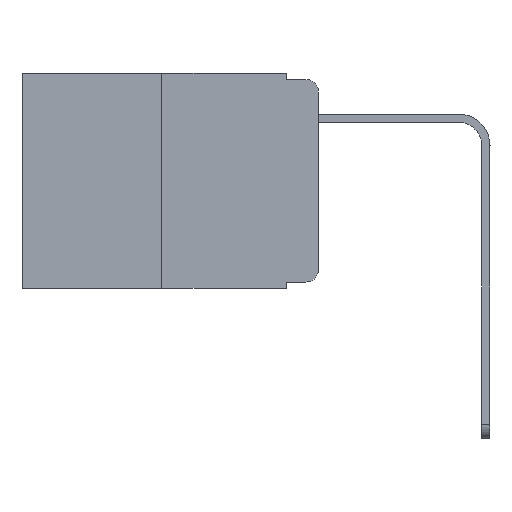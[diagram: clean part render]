
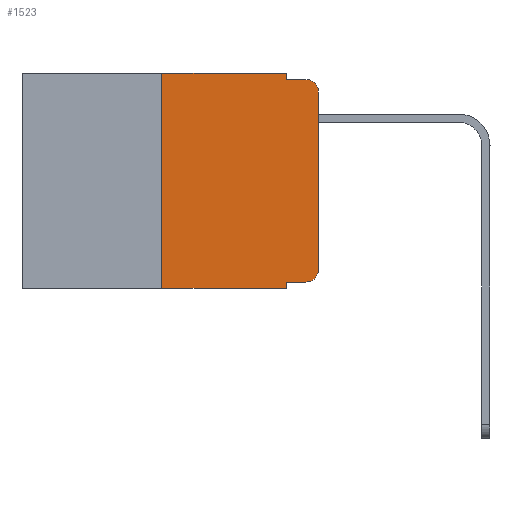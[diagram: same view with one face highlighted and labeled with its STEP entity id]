
A CAD part, left-side view. The second image highlights one B-rep face of the part: STEP entity #1523.
In plain terms, the highlighted planar face has unit normal (-1, 0, 0).
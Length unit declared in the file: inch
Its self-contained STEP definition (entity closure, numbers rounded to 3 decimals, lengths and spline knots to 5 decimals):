
#162 = CARTESIAN_POINT ( 'NONE',  ( 0., 0.473, 0. ) ) ;
#573 = CARTESIAN_POINT ( 'NONE',  ( 0., 0.473, -0.343 ) ) ;
#917 = EDGE_CURVE ( 'NONE', #14089, #12298, #3522, .T. ) ;
#1089 = VERTEX_POINT ( 'NONE', #14140 ) ;
#1265 = ORIENTED_EDGE ( 'NONE', *, *, #12177, .T. ) ;
#1493 = VERTEX_POINT ( 'NONE', #6013 ) ;
#1523 = ADVANCED_FACE ( 'NONE', ( #13903 ), #1693, .F. ) ;
#1693 = PLANE ( 'NONE',  #10979 ) ;
#1792 = CIRCLE ( 'NONE', #14482, 0.02 ) ;
#2038 = ORIENTED_EDGE ( 'NONE', *, *, #14747, .F. ) ;
#2066 = CARTESIAN_POINT ( 'NONE',  ( 0., 0.02, -0.313 ) ) ;
#2218 = VECTOR ( 'NONE', #8968, 39.37008 ) ;
#3108 = DIRECTION ( 'NONE',  ( 0., 0., -1. ) ) ;
#3147 = CARTESIAN_POINT ( 'NONE',  ( 0., 0.051, 0. ) ) ;
#3240 = DIRECTION ( 'NONE',  ( -1., 0., 0. ) ) ;
#3414 = VECTOR ( 'NONE', #8670, 39.37008 ) ;
#3522 = LINE ( 'NONE', #4336, #13734 ) ;
#3771 = LINE ( 'NONE', #573, #10218 ) ;
#3884 = VERTEX_POINT ( 'NONE', #7558 ) ;
#3907 = ORIENTED_EDGE ( 'NONE', *, *, #4260, .F. ) ;
#4260 = EDGE_CURVE ( 'NONE', #9914, #3884, #13710, .T. ) ;
#4336 = CARTESIAN_POINT ( 'NONE',  ( 0., 0., 0. ) ) ;
#4517 = DIRECTION ( 'NONE',  ( 0., 0., 1. ) ) ;
#5112 = LINE ( 'NONE', #3147, #7447 ) ;
#5507 = ORIENTED_EDGE ( 'NONE', *, *, #7386, .T. ) ;
#5905 = EDGE_CURVE ( 'NONE', #3884, #1493, #5112, .T. ) ;
#6013 = CARTESIAN_POINT ( 'NONE',  ( 0., 0.051, -0.01 ) ) ;
#6041 = CARTESIAN_POINT ( 'NONE',  ( 0., 0.25, 0. ) ) ;
#6193 = EDGE_CURVE ( 'NONE', #1493, #10311, #9038, .T. ) ;
#6269 = DIRECTION ( 'NONE',  ( -1., 0., 0. ) ) ;
#6521 = DIRECTION ( 'NONE',  ( 0., 0., -1. ) ) ;
#6540 = ORIENTED_EDGE ( 'NONE', *, *, #12832, .T. ) ;
#7133 = ORIENTED_EDGE ( 'NONE', *, *, #8048, .T. ) ;
#7386 = EDGE_CURVE ( 'NONE', #1089, #9643, #7921, .T. ) ;
#7447 = VECTOR ( 'NONE', #14461, 39.37008 ) ;
#7510 = CARTESIAN_POINT ( 'NONE',  ( 0., 0., -0.03 ) ) ;
#7558 = CARTESIAN_POINT ( 'NONE',  ( 0., 0.051, 0. ) ) ;
#7658 = CARTESIAN_POINT ( 'NONE',  ( 0., 0.051, -0.333 ) ) ;
#7764 = CARTESIAN_POINT ( 'NONE',  ( 0., 0.25, 0. ) ) ;
#7782 = VECTOR ( 'NONE', #9279, 39.37008 ) ;
#7921 = LINE ( 'NONE', #7658, #2218 ) ;
#8048 = EDGE_CURVE ( 'NONE', #9643, #14089, #14553, .T. ) ;
#8395 = CARTESIAN_POINT ( 'NONE',  ( 0., 0.25, -0.343 ) ) ;
#8418 = CARTESIAN_POINT ( 'NONE',  ( 0., 0.02, -0.01 ) ) ;
#8670 = DIRECTION ( 'NONE',  ( 0., 0., -1. ) ) ;
#8880 = ORIENTED_EDGE ( 'NONE', *, *, #13408, .F. ) ;
#8968 = DIRECTION ( 'NONE',  ( 0., -1., 0. ) ) ;
#9038 = LINE ( 'NONE', #11573, #7782 ) ;
#9122 = CARTESIAN_POINT ( 'NONE',  ( 0., 0.051, -0.343 ) ) ;
#9279 = DIRECTION ( 'NONE',  ( 0., -1., 0. ) ) ;
#9422 = VECTOR ( 'NONE', #13908, 39.37008 ) ;
#9643 = VERTEX_POINT ( 'NONE', #10769 ) ;
#9914 = VERTEX_POINT ( 'NONE', #7764 ) ;
#10009 = ORIENTED_EDGE ( 'NONE', *, *, #6193, .F. ) ;
#10218 = VECTOR ( 'NONE', #12056, 39.37008 ) ;
#10311 = VERTEX_POINT ( 'NONE', #8418 ) ;
#10760 = AXIS2_PLACEMENT_3D ( 'NONE', #2066, #3240, #3108 ) ;
#10769 = CARTESIAN_POINT ( 'NONE',  ( 0., 0.02, -0.333 ) ) ;
#10979 = AXIS2_PLACEMENT_3D ( 'NONE', #12221, #13377, #6521 ) ;
#11573 = CARTESIAN_POINT ( 'NONE',  ( 0., 0.051, -0.01 ) ) ;
#11784 = LINE ( 'NONE', #6041, #13391 ) ;
#12056 = DIRECTION ( 'NONE',  ( 0., -1., 0. ) ) ;
#12071 = CARTESIAN_POINT ( 'NONE',  ( 0., 0., -0.313 ) ) ;
#12106 = CARTESIAN_POINT ( 'NONE',  ( 0., 0.051, 0. ) ) ;
#12140 = EDGE_LOOP ( 'NONE', ( #13094, #6540, #10009, #13358, #3907, #8880, #1265, #2038, #5507, #7133 ) ) ;
#12177 = EDGE_CURVE ( 'NONE', #13270, #14366, #3771, .T. ) ;
#12221 = CARTESIAN_POINT ( 'NONE',  ( 0., 0.473, 0. ) ) ;
#12298 = VERTEX_POINT ( 'NONE', #7510 ) ;
#12362 = LINE ( 'NONE', #12106, #3414 ) ;
#12832 = EDGE_CURVE ( 'NONE', #12298, #10311, #1792, .T. ) ;
#13010 = CARTESIAN_POINT ( 'NONE',  ( 0., 0.02, -0.03 ) ) ;
#13094 = ORIENTED_EDGE ( 'NONE', *, *, #917, .T. ) ;
#13270 = VERTEX_POINT ( 'NONE', #8395 ) ;
#13358 = ORIENTED_EDGE ( 'NONE', *, *, #5905, .F. ) ;
#13377 = DIRECTION ( 'NONE',  ( 1., 0., 0. ) ) ;
#13391 = VECTOR ( 'NONE', #13993, 39.37008 ) ;
#13408 = EDGE_CURVE ( 'NONE', #13270, #9914, #11784, .T. ) ;
#13710 = LINE ( 'NONE', #162, #9422 ) ;
#13734 = VECTOR ( 'NONE', #4517, 39.37008 ) ;
#13903 = FACE_OUTER_BOUND ( 'NONE', #12140, .T. ) ;
#13908 = DIRECTION ( 'NONE',  ( 0., -1., 0. ) ) ;
#13993 = DIRECTION ( 'NONE',  ( 0., 0., 1. ) ) ;
#14089 = VERTEX_POINT ( 'NONE', #12071 ) ;
#14140 = CARTESIAN_POINT ( 'NONE',  ( 0., 0.051, -0.333 ) ) ;
#14270 = DIRECTION ( 'NONE',  ( 0., 0., -1. ) ) ;
#14366 = VERTEX_POINT ( 'NONE', #9122 ) ;
#14461 = DIRECTION ( 'NONE',  ( 0., 0., -1. ) ) ;
#14482 = AXIS2_PLACEMENT_3D ( 'NONE', #13010, #6269, #14270 ) ;
#14553 = CIRCLE ( 'NONE', #10760, 0.02 ) ;
#14747 = EDGE_CURVE ( 'NONE', #1089, #14366, #12362, .T. ) ;
